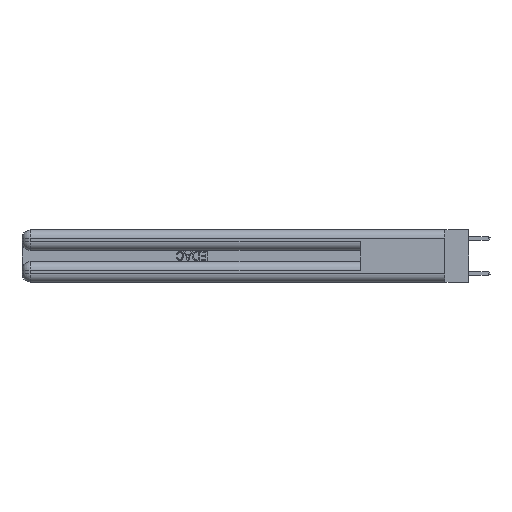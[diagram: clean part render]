
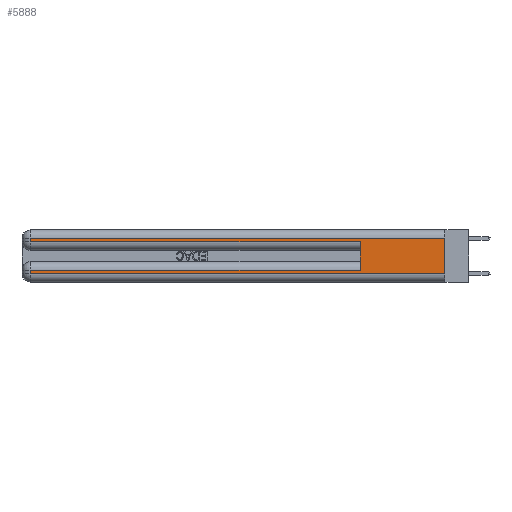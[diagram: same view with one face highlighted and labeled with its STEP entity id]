
A CAD part, left-side view. The second image highlights one B-rep face of the part: STEP entity #5888.
In plain terms, the highlighted planar face has unit normal (-1, 0, 0).
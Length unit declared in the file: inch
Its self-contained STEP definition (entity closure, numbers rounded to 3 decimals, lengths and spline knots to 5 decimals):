
#161 = CARTESIAN_POINT ( 'NONE',  ( 0., 2.94, 0.37 ) ) ;
#215 = DIRECTION ( 'NONE',  ( 0., 0., -1. ) ) ;
#593 = ORIENTED_EDGE ( 'NONE', *, *, #8542, .T. ) ;
#815 = ORIENTED_EDGE ( 'NONE', *, *, #3656, .T. ) ;
#1514 = CARTESIAN_POINT ( 'NONE',  ( 0., 0.6, 0.085 ) ) ;
#1522 = EDGE_CURVE ( 'NONE', #25298, #20833, #6013, .T. ) ;
#1559 = ORIENTED_EDGE ( 'NONE', *, *, #4545, .T. ) ;
#2110 = PLANE ( 'NONE',  #8708 ) ;
#2166 = CARTESIAN_POINT ( 'NONE',  ( 0., 0., 0.285 ) ) ;
#3126 = VECTOR ( 'NONE', #23084, 39.37008 ) ;
#3656 = EDGE_CURVE ( 'NONE', #23963, #20833, #22658, .T. ) ;
#3782 = LINE ( 'NONE', #22244, #8752 ) ;
#4517 = EDGE_CURVE ( 'NONE', #18123, #11976, #22971, .T. ) ;
#4545 = EDGE_CURVE ( 'NONE', #11976, #23963, #24816, .T. ) ;
#4831 = ORIENTED_EDGE ( 'NONE', *, *, #13406, .T. ) ;
#5230 = ORIENTED_EDGE ( 'NONE', *, *, #4517, .T. ) ;
#5888 = ADVANCED_FACE ( 'NONE', ( #8563 ), #2110, .F. ) ;
#6013 = LINE ( 'NONE', #8051, #6331 ) ;
#6331 = VECTOR ( 'NONE', #22490, 39.37008 ) ;
#6506 = VECTOR ( 'NONE', #16516, 39.37008 ) ;
#6566 = VECTOR ( 'NONE', #215, 39.37008 ) ;
#6637 = DIRECTION ( 'NONE',  ( 0., 1., 0. ) ) ;
#6770 = CARTESIAN_POINT ( 'NONE',  ( 0., 0., 0.31 ) ) ;
#6804 = CARTESIAN_POINT ( 'NONE',  ( 0., 2.94, 0.31 ) ) ;
#6984 = ORIENTED_EDGE ( 'NONE', *, *, #1522, .F. ) ;
#7049 = EDGE_CURVE ( 'NONE', #18123, #15913, #3782, .T. ) ;
#7791 = VERTEX_POINT ( 'NONE', #8701 ) ;
#8051 = CARTESIAN_POINT ( 'NONE',  ( 0., 0.6, 0.145 ) ) ;
#8360 = DIRECTION ( 'NONE',  ( 0., 0., -1. ) ) ;
#8529 = CARTESIAN_POINT ( 'NONE',  ( 0., 2.94, 0.37 ) ) ;
#8542 = EDGE_CURVE ( 'NONE', #23185, #7791, #10599, .T. ) ;
#8563 = FACE_OUTER_BOUND ( 'NONE', #14811, .T. ) ;
#8701 = CARTESIAN_POINT ( 'NONE',  ( 0., 2.94, 0.06 ) ) ;
#8708 = AXIS2_PLACEMENT_3D ( 'NONE', #20855, #12317, #10288 ) ;
#8752 = VECTOR ( 'NONE', #25878, 39.37008 ) ;
#8797 = CARTESIAN_POINT ( 'NONE',  ( 0., 0.6, 0.285 ) ) ;
#10229 = CARTESIAN_POINT ( 'NONE',  ( 0., 0., 0.31 ) ) ;
#10288 = DIRECTION ( 'NONE',  ( 0., 0., -1. ) ) ;
#10599 = LINE ( 'NONE', #161, #13427 ) ;
#11334 = ORIENTED_EDGE ( 'NONE', *, *, #21308, .T. ) ;
#11976 = VERTEX_POINT ( 'NONE', #6804 ) ;
#12317 = DIRECTION ( 'NONE',  ( 1., 0., 0. ) ) ;
#13406 = EDGE_CURVE ( 'NONE', #25298, #23185, #24947, .T. ) ;
#13427 = VECTOR ( 'NONE', #8360, 39.37008 ) ;
#13545 = CARTESIAN_POINT ( 'NONE',  ( 0., 2.94, 0.285 ) ) ;
#14754 = DIRECTION ( 'NONE',  ( 0., -1., 0. ) ) ;
#14811 = EDGE_LOOP ( 'NONE', ( #26372, #5230, #1559, #815, #6984, #4831, #593, #11334 ) ) ;
#15913 = VERTEX_POINT ( 'NONE', #22596 ) ;
#16273 = CARTESIAN_POINT ( 'NONE',  ( 0., 2.94, 0.085 ) ) ;
#16516 = DIRECTION ( 'NONE',  ( 0., -1., 0. ) ) ;
#17158 = CARTESIAN_POINT ( 'NONE',  ( 0., 0., 0.085 ) ) ;
#18123 = VERTEX_POINT ( 'NONE', #10229 ) ;
#18375 = CARTESIAN_POINT ( 'NONE',  ( 0., 0., 0.06 ) ) ;
#20440 = VECTOR ( 'NONE', #14754, 39.37008 ) ;
#20833 = VERTEX_POINT ( 'NONE', #8797 ) ;
#20855 = CARTESIAN_POINT ( 'NONE',  ( 0., 0., 0.37 ) ) ;
#21308 = EDGE_CURVE ( 'NONE', #7791, #15913, #24918, .T. ) ;
#21644 = VECTOR ( 'NONE', #6637, 39.37008 ) ;
#22244 = CARTESIAN_POINT ( 'NONE',  ( 0., 0., 0.37 ) ) ;
#22490 = DIRECTION ( 'NONE',  ( 0., 0., 1. ) ) ;
#22596 = CARTESIAN_POINT ( 'NONE',  ( 0., 0., 0.06 ) ) ;
#22658 = LINE ( 'NONE', #2166, #20440 ) ;
#22971 = LINE ( 'NONE', #6770, #3126 ) ;
#23084 = DIRECTION ( 'NONE',  ( 0., 1., 0. ) ) ;
#23185 = VERTEX_POINT ( 'NONE', #16273 ) ;
#23963 = VERTEX_POINT ( 'NONE', #13545 ) ;
#24816 = LINE ( 'NONE', #8529, #6566 ) ;
#24918 = LINE ( 'NONE', #18375, #6506 ) ;
#24947 = LINE ( 'NONE', #17158, #21644 ) ;
#25298 = VERTEX_POINT ( 'NONE', #1514 ) ;
#25878 = DIRECTION ( 'NONE',  ( 0., 0., -1. ) ) ;
#26372 = ORIENTED_EDGE ( 'NONE', *, *, #7049, .F. ) ;
